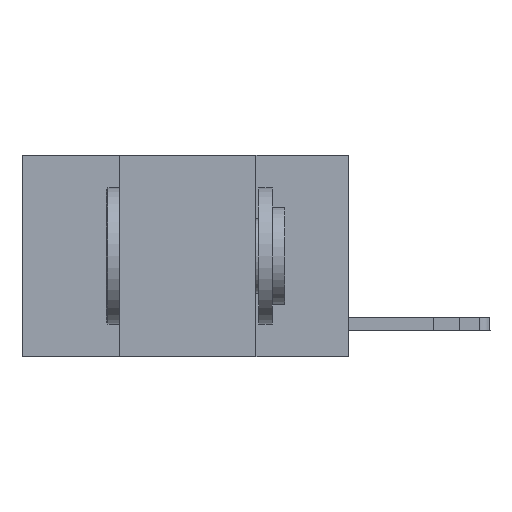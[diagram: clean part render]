
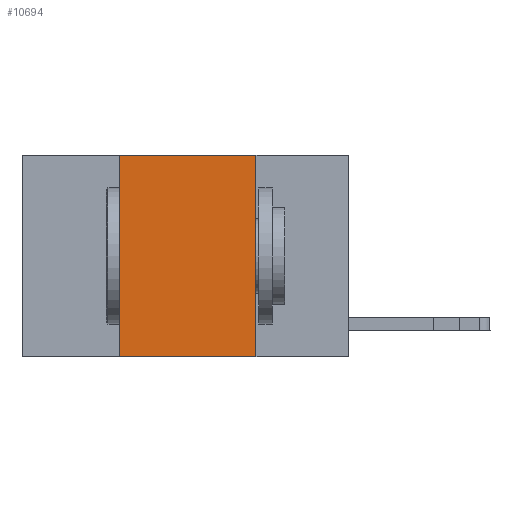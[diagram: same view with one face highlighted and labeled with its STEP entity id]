
A CAD part, left-side view. The second image highlights one B-rep face of the part: STEP entity #10694.
In plain terms, the highlighted planar face has unit normal (-1, 0, 0).
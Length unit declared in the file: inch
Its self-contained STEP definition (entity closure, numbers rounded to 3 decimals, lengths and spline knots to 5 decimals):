
#170 = LINE ( 'NONE', #13224, #10714 ) ;
#199 = EDGE_CURVE ( 'NONE', #8991, #23923, #21441, .T. ) ;
#242 = DIRECTION ( 'NONE',  ( 0., 0., 1. ) ) ;
#1133 = AXIS2_PLACEMENT_3D ( 'NONE', #20380, #11419, #1180 ) ;
#1180 = DIRECTION ( 'NONE',  ( 0., 0., -1. ) ) ;
#1769 = VERTEX_POINT ( 'NONE', #5185 ) ;
#4528 = ORIENTED_EDGE ( 'NONE', *, *, #199, .F. ) ;
#4662 = FACE_OUTER_BOUND ( 'NONE', #7843, .T. ) ;
#4794 = EDGE_CURVE ( 'NONE', #23923, #16983, #170, .T. ) ;
#5185 = CARTESIAN_POINT ( 'NONE',  ( 0., 0.17, -0.37 ) ) ;
#7843 = EDGE_LOOP ( 'NONE', ( #25290, #18612, #4528, #7915 ) ) ;
#7915 = ORIENTED_EDGE ( 'NONE', *, *, #24670, .T. ) ;
#8249 = LINE ( 'NONE', #12336, #12685 ) ;
#8712 = DIRECTION ( 'NONE',  ( 0., -1., 0. ) ) ;
#8818 = CARTESIAN_POINT ( 'NONE',  ( 0., 0.6, -0.37 ) ) ;
#8991 = VERTEX_POINT ( 'NONE', #16047 ) ;
#10694 = ADVANCED_FACE ( 'NONE', ( #4662 ), #13250, .F. ) ;
#10714 = VECTOR ( 'NONE', #8712, 39.37008 ) ;
#11419 = DIRECTION ( 'NONE',  ( 1., 0., 0. ) ) ;
#12336 = CARTESIAN_POINT ( 'NONE',  ( 0., 0.17, 0. ) ) ;
#12685 = VECTOR ( 'NONE', #20892, 39.37008 ) ;
#13224 = CARTESIAN_POINT ( 'NONE',  ( 0., 0.6, 0. ) ) ;
#13250 = PLANE ( 'NONE',  #1133 ) ;
#14569 = DIRECTION ( 'NONE',  ( 0., -1., 0. ) ) ;
#14979 = LINE ( 'NONE', #8818, #26278 ) ;
#16047 = CARTESIAN_POINT ( 'NONE',  ( 0., 0.42, -0.37 ) ) ;
#16983 = VERTEX_POINT ( 'NONE', #27230 ) ;
#17484 = CARTESIAN_POINT ( 'NONE',  ( 0., 0.42, 0. ) ) ;
#18612 = ORIENTED_EDGE ( 'NONE', *, *, #4794, .F. ) ;
#20298 = EDGE_CURVE ( 'NONE', #16983, #1769, #8249, .T. ) ;
#20380 = CARTESIAN_POINT ( 'NONE',  ( 0., 0.6, 0. ) ) ;
#20892 = DIRECTION ( 'NONE',  ( 0., 0., -1. ) ) ;
#21441 = LINE ( 'NONE', #17484, #26383 ) ;
#23923 = VERTEX_POINT ( 'NONE', #27660 ) ;
#24670 = EDGE_CURVE ( 'NONE', #8991, #1769, #14979, .T. ) ;
#25290 = ORIENTED_EDGE ( 'NONE', *, *, #20298, .F. ) ;
#26278 = VECTOR ( 'NONE', #14569, 39.37008 ) ;
#26383 = VECTOR ( 'NONE', #242, 39.37008 ) ;
#27230 = CARTESIAN_POINT ( 'NONE',  ( 0., 0.17, 0. ) ) ;
#27660 = CARTESIAN_POINT ( 'NONE',  ( 0., 0.42, 0. ) ) ;
